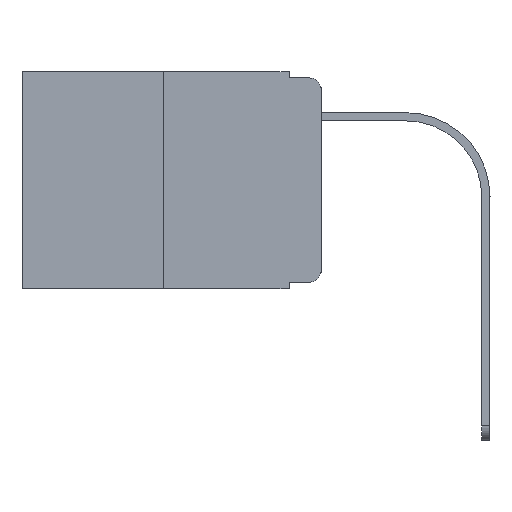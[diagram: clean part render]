
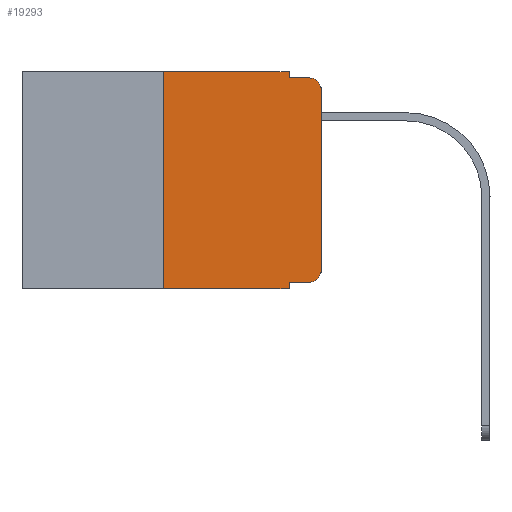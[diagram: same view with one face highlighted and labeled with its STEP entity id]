
A CAD part, left-side view. The second image highlights one B-rep face of the part: STEP entity #19293.
In plain terms, the highlighted planar face has unit normal (-1, 0, 0).
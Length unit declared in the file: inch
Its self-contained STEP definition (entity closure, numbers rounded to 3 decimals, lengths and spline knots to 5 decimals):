
#648 = VERTEX_POINT ( 'NONE', #8064 ) ;
#700 = VECTOR ( 'NONE', #20379, 39.37008 ) ;
#881 = DIRECTION ( 'NONE',  ( 0., 0., -1. ) ) ;
#894 = CARTESIAN_POINT ( 'NONE',  ( 0., 0.051, 0. ) ) ;
#1223 = FACE_OUTER_BOUND ( 'NONE', #4397, .T. ) ;
#1258 = ORIENTED_EDGE ( 'NONE', *, *, #16839, .F. ) ;
#1342 = EDGE_CURVE ( 'NONE', #10337, #19401, #6446, .T. ) ;
#1546 = CARTESIAN_POINT ( 'NONE',  ( 0., 0.02, -0.01 ) ) ;
#1582 = ORIENTED_EDGE ( 'NONE', *, *, #6027, .T. ) ;
#1983 = CARTESIAN_POINT ( 'NONE',  ( 0., 0.051, -0.01 ) ) ;
#2652 = CARTESIAN_POINT ( 'NONE',  ( 0., 0.051, -0.01 ) ) ;
#2778 = VECTOR ( 'NONE', #14170, 39.37008 ) ;
#2883 = EDGE_CURVE ( 'NONE', #17528, #648, #3199, .T. ) ;
#2956 = DIRECTION ( 'NONE',  ( 0., 0., -1. ) ) ;
#3018 = VECTOR ( 'NONE', #2956, 39.37008 ) ;
#3058 = DIRECTION ( 'NONE',  ( -1., 0., 0. ) ) ;
#3146 = EDGE_CURVE ( 'NONE', #8520, #648, #6240, .T. ) ;
#3162 = CARTESIAN_POINT ( 'NONE',  ( 0., 0.051, -0.333 ) ) ;
#3199 = LINE ( 'NONE', #6928, #18725 ) ;
#4137 = CARTESIAN_POINT ( 'NONE',  ( 0., 0., 0. ) ) ;
#4397 = EDGE_LOOP ( 'NONE', ( #17728, #4607, #1258, #17708, #18119, #18623, #9613, #14848, #1582, #8444 ) ) ;
#4606 = VERTEX_POINT ( 'NONE', #11030 ) ;
#4607 = ORIENTED_EDGE ( 'NONE', *, *, #1342, .T. ) ;
#4839 = LINE ( 'NONE', #6086, #700 ) ;
#4987 = AXIS2_PLACEMENT_3D ( 'NONE', #6159, #9370, #21726 ) ;
#5543 = EDGE_CURVE ( 'NONE', #4606, #10337, #21953, .T. ) ;
#5710 = CIRCLE ( 'NONE', #10077, 0.02 ) ;
#6027 = EDGE_CURVE ( 'NONE', #8520, #10702, #14068, .T. ) ;
#6086 = CARTESIAN_POINT ( 'NONE',  ( 0., 0.473, 0. ) ) ;
#6159 = CARTESIAN_POINT ( 'NONE',  ( 0., 0.02, -0.03 ) ) ;
#6240 = LINE ( 'NONE', #894, #3018 ) ;
#6274 = DIRECTION ( 'NONE',  ( 0., 0., 1. ) ) ;
#6446 = CIRCLE ( 'NONE', #4987, 0.02 ) ;
#6488 = EDGE_CURVE ( 'NONE', #8110, #17467, #15733, .T. ) ;
#6592 = EDGE_CURVE ( 'NONE', #17528, #7401, #13107, .T. ) ;
#6928 = CARTESIAN_POINT ( 'NONE',  ( 0., 0.473, -0.343 ) ) ;
#6938 = DIRECTION ( 'NONE',  ( 0., 0., -1. ) ) ;
#6990 = DIRECTION ( 'NONE',  ( 0., -1., 0. ) ) ;
#7401 = VERTEX_POINT ( 'NONE', #11345 ) ;
#8064 = CARTESIAN_POINT ( 'NONE',  ( 0., 0.051, -0.343 ) ) ;
#8110 = VERTEX_POINT ( 'NONE', #13472 ) ;
#8138 = VECTOR ( 'NONE', #6938, 39.37008 ) ;
#8444 = ORIENTED_EDGE ( 'NONE', *, *, #16297, .T. ) ;
#8465 = LINE ( 'NONE', #1983, #2778 ) ;
#8520 = VERTEX_POINT ( 'NONE', #3162 ) ;
#8807 = VECTOR ( 'NONE', #6274, 39.37008 ) ;
#9370 = DIRECTION ( 'NONE',  ( -1., 0., 0. ) ) ;
#9613 = ORIENTED_EDGE ( 'NONE', *, *, #2883, .T. ) ;
#10077 = AXIS2_PLACEMENT_3D ( 'NONE', #11715, #3058, #20192 ) ;
#10139 = DIRECTION ( 'NONE',  ( 0., -1., 0. ) ) ;
#10152 = EDGE_CURVE ( 'NONE', #7401, #8110, #4839, .T. ) ;
#10337 = VERTEX_POINT ( 'NONE', #17814 ) ;
#10702 = VERTEX_POINT ( 'NONE', #13456 ) ;
#11030 = CARTESIAN_POINT ( 'NONE',  ( 0., 0., -0.313 ) ) ;
#11345 = CARTESIAN_POINT ( 'NONE',  ( 0., 0.25, 0. ) ) ;
#11399 = CARTESIAN_POINT ( 'NONE',  ( 0., 0.25, 0. ) ) ;
#11715 = CARTESIAN_POINT ( 'NONE',  ( 0., 0.02, -0.313 ) ) ;
#13107 = LINE ( 'NONE', #11399, #20204 ) ;
#13456 = CARTESIAN_POINT ( 'NONE',  ( 0., 0.02, -0.333 ) ) ;
#13472 = CARTESIAN_POINT ( 'NONE',  ( 0., 0.051, 0. ) ) ;
#13543 = CARTESIAN_POINT ( 'NONE',  ( 0., 0.25, -0.343 ) ) ;
#14068 = LINE ( 'NONE', #17400, #18711 ) ;
#14125 = CARTESIAN_POINT ( 'NONE',  ( 0., 0.051, 0. ) ) ;
#14170 = DIRECTION ( 'NONE',  ( 0., -1., 0. ) ) ;
#14848 = ORIENTED_EDGE ( 'NONE', *, *, #3146, .F. ) ;
#15014 = DIRECTION ( 'NONE',  ( 1., 0., 0. ) ) ;
#15127 = CARTESIAN_POINT ( 'NONE',  ( 0., 0.473, 0. ) ) ;
#15733 = LINE ( 'NONE', #14125, #8138 ) ;
#16297 = EDGE_CURVE ( 'NONE', #10702, #4606, #5710, .T. ) ;
#16421 = DIRECTION ( 'NONE',  ( 0., 0., 1. ) ) ;
#16839 = EDGE_CURVE ( 'NONE', #17467, #19401, #8465, .T. ) ;
#17400 = CARTESIAN_POINT ( 'NONE',  ( 0., 0.051, -0.333 ) ) ;
#17467 = VERTEX_POINT ( 'NONE', #2652 ) ;
#17528 = VERTEX_POINT ( 'NONE', #13543 ) ;
#17708 = ORIENTED_EDGE ( 'NONE', *, *, #6488, .F. ) ;
#17728 = ORIENTED_EDGE ( 'NONE', *, *, #5543, .T. ) ;
#17814 = CARTESIAN_POINT ( 'NONE',  ( 0., 0., -0.03 ) ) ;
#18119 = ORIENTED_EDGE ( 'NONE', *, *, #10152, .F. ) ;
#18581 = PLANE ( 'NONE',  #21420 ) ;
#18623 = ORIENTED_EDGE ( 'NONE', *, *, #6592, .F. ) ;
#18711 = VECTOR ( 'NONE', #6990, 39.37008 ) ;
#18725 = VECTOR ( 'NONE', #10139, 39.37008 ) ;
#19293 = ADVANCED_FACE ( 'NONE', ( #1223 ), #18581, .F. ) ;
#19401 = VERTEX_POINT ( 'NONE', #1546 ) ;
#20192 = DIRECTION ( 'NONE',  ( 0., 0., -1. ) ) ;
#20204 = VECTOR ( 'NONE', #16421, 39.37008 ) ;
#20379 = DIRECTION ( 'NONE',  ( 0., -1., 0. ) ) ;
#21420 = AXIS2_PLACEMENT_3D ( 'NONE', #15127, #15014, #881 ) ;
#21726 = DIRECTION ( 'NONE',  ( 0., 0., -1. ) ) ;
#21953 = LINE ( 'NONE', #4137, #8807 ) ;
